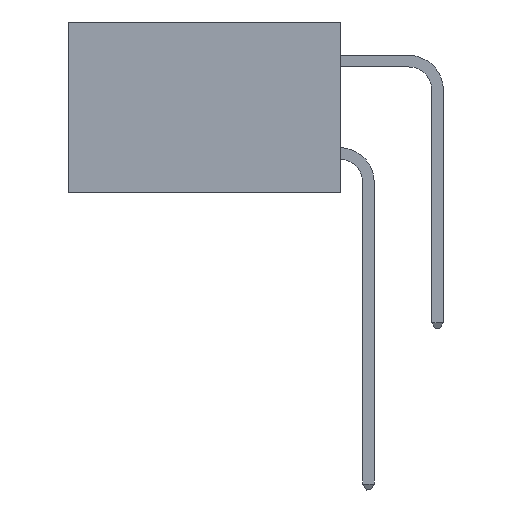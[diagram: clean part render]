
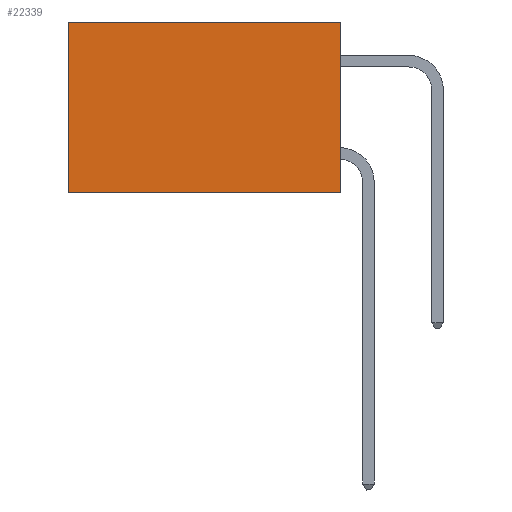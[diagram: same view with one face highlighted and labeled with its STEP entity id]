
A CAD part, left-side view. The second image highlights one B-rep face of the part: STEP entity #22339.
In plain terms, the highlighted planar face has unit normal (-1, 0, 0).
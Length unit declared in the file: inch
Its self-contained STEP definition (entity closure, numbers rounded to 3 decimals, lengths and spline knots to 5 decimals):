
#172 = FACE_OUTER_BOUND ( 'NONE', #19470, .T. ) ;
#357 = DIRECTION ( 'NONE',  ( 1., 0., 0. ) ) ;
#896 = DIRECTION ( 'NONE',  ( 0., 1., 0. ) ) ;
#2276 = ORIENTED_EDGE ( 'NONE', *, *, #20065, .T. ) ;
#2328 = ORIENTED_EDGE ( 'NONE', *, *, #20513, .F. ) ;
#2520 = ORIENTED_EDGE ( 'NONE', *, *, #22824, .F. ) ;
#2542 = ORIENTED_EDGE ( 'NONE', *, *, #10091, .T. ) ;
#5015 = VERTEX_POINT ( 'NONE', #11096 ) ;
#5296 = LINE ( 'NONE', #17148, #13703 ) ;
#5314 = LINE ( 'NONE', #19527, #10124 ) ;
#5425 = DIRECTION ( 'NONE',  ( 0., 0., -1. ) ) ;
#6850 = VECTOR ( 'NONE', #896, 39.37008 ) ;
#7433 = LINE ( 'NONE', #15422, #6850 ) ;
#8896 = LINE ( 'NONE', #12555, #13051 ) ;
#8911 = DIRECTION ( 'NONE',  ( 0., 0., -1. ) ) ;
#9460 = CARTESIAN_POINT ( 'NONE',  ( 0.277, 0., -0.37 ) ) ;
#10091 = EDGE_CURVE ( 'NONE', #5015, #13795, #7433, .T. ) ;
#10124 = VECTOR ( 'NONE', #8911, 39.37008 ) ;
#11096 = CARTESIAN_POINT ( 'NONE',  ( 0.277, 0., 0. ) ) ;
#11384 = PLANE ( 'NONE',  #16509 ) ;
#12555 = CARTESIAN_POINT ( 'NONE',  ( 0.277, 0., -0.37 ) ) ;
#13051 = VECTOR ( 'NONE', #5425, 39.37008 ) ;
#13157 = DIRECTION ( 'NONE',  ( 0., 0., -1. ) ) ;
#13262 = CARTESIAN_POINT ( 'NONE',  ( 0.277, 0.59, -0.37 ) ) ;
#13703 = VECTOR ( 'NONE', #18954, 39.37008 ) ;
#13795 = VERTEX_POINT ( 'NONE', #16744 ) ;
#15422 = CARTESIAN_POINT ( 'NONE',  ( 0.277, 0., 0. ) ) ;
#16509 = AXIS2_PLACEMENT_3D ( 'NONE', #21931, #357, #13157 ) ;
#16744 = CARTESIAN_POINT ( 'NONE',  ( 0.277, 0.59, 0. ) ) ;
#17148 = CARTESIAN_POINT ( 'NONE',  ( 0.277, 0., -0.37 ) ) ;
#18954 = DIRECTION ( 'NONE',  ( 0., 1., 0. ) ) ;
#19470 = EDGE_LOOP ( 'NONE', ( #2276, #2328, #2520, #2542 ) ) ;
#19527 = CARTESIAN_POINT ( 'NONE',  ( 0.277, 0.59, -0.37 ) ) ;
#19732 = VERTEX_POINT ( 'NONE', #9460 ) ;
#20065 = EDGE_CURVE ( 'NONE', #13795, #21747, #5314, .T. ) ;
#20513 = EDGE_CURVE ( 'NONE', #19732, #21747, #5296, .T. ) ;
#21747 = VERTEX_POINT ( 'NONE', #13262 ) ;
#21931 = CARTESIAN_POINT ( 'NONE',  ( 0.277, 0., -0.37 ) ) ;
#22339 = ADVANCED_FACE ( 'NONE', ( #172 ), #11384, .F. ) ;
#22824 = EDGE_CURVE ( 'NONE', #5015, #19732, #8896, .T. ) ;
